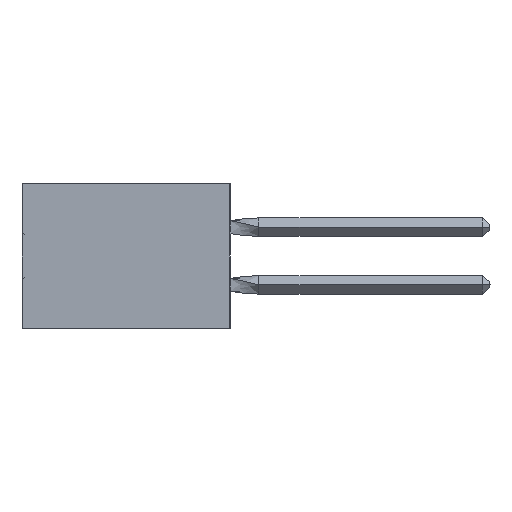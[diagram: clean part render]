
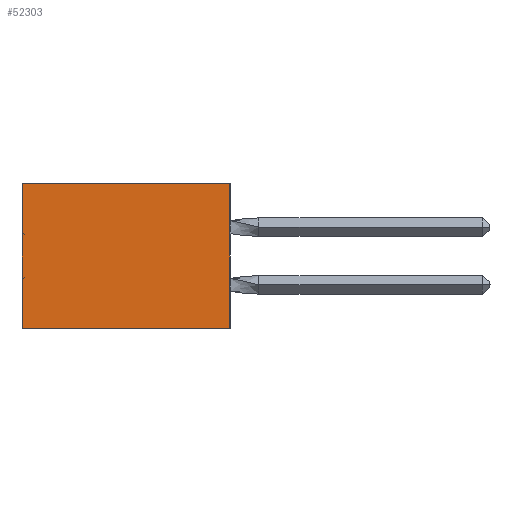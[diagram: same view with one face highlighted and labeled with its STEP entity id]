
A CAD part, left-side view. The second image highlights one B-rep face of the part: STEP entity #52303.
In plain terms, the highlighted planar face has unit normal (-1, 0, 0).
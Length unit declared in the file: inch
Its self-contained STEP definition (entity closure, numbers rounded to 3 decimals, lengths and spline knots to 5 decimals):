
#1045 = CARTESIAN_POINT ( 'NONE',  ( 0.305, 0., -0.5 ) ) ;
#2218 = ORIENTED_EDGE ( 'NONE', *, *, #22151, .T. ) ;
#2652 = FACE_OUTER_BOUND ( 'NONE', #12674, .T. ) ;
#3414 = ORIENTED_EDGE ( 'NONE', *, *, #12335, .F. ) ;
#4339 = EDGE_CURVE ( 'NONE', #31981, #32026, #5787, .T. ) ;
#4480 = LINE ( 'NONE', #23411, #48323 ) ;
#5787 = LINE ( 'NONE', #17353, #41653 ) ;
#7700 = VERTEX_POINT ( 'NONE', #12366 ) ;
#9683 = LINE ( 'NONE', #1045, #44156 ) ;
#11060 = CARTESIAN_POINT ( 'NONE',  ( 0.305, 0., -0.5 ) ) ;
#12187 = DIRECTION ( 'NONE',  ( 1., 0., 0. ) ) ;
#12335 = EDGE_CURVE ( 'NONE', #7700, #26019, #39653, .T. ) ;
#12366 = CARTESIAN_POINT ( 'NONE',  ( 0.305, 0., 0. ) ) ;
#12674 = EDGE_LOOP ( 'NONE', ( #26959, #19417, #3414, #2218 ) ) ;
#12756 = PLANE ( 'NONE',  #18285 ) ;
#17353 = CARTESIAN_POINT ( 'NONE',  ( 0.305, 0.72, -0.5 ) ) ;
#17668 = CARTESIAN_POINT ( 'NONE',  ( 0.305, 0.72, 0. ) ) ;
#18285 = AXIS2_PLACEMENT_3D ( 'NONE', #42452, #12187, #38009 ) ;
#19417 = ORIENTED_EDGE ( 'NONE', *, *, #46550, .F. ) ;
#22151 = EDGE_CURVE ( 'NONE', #7700, #31981, #4480, .T. ) ;
#23411 = CARTESIAN_POINT ( 'NONE',  ( 0.305, 0., 0. ) ) ;
#26019 = VERTEX_POINT ( 'NONE', #11060 ) ;
#26959 = ORIENTED_EDGE ( 'NONE', *, *, #4339, .T. ) ;
#31131 = DIRECTION ( 'NONE',  ( 0., 1., 0. ) ) ;
#31981 = VERTEX_POINT ( 'NONE', #17668 ) ;
#32026 = VERTEX_POINT ( 'NONE', #35929 ) ;
#35929 = CARTESIAN_POINT ( 'NONE',  ( 0.305, 0.72, -0.5 ) ) ;
#37259 = DIRECTION ( 'NONE',  ( 0., 0., -1. ) ) ;
#38009 = DIRECTION ( 'NONE',  ( 0., 0., -1. ) ) ;
#39653 = LINE ( 'NONE', #45962, #44252 ) ;
#41653 = VECTOR ( 'NONE', #51001, 39.37008 ) ;
#42452 = CARTESIAN_POINT ( 'NONE',  ( 0.305, 0., -0.5 ) ) ;
#44156 = VECTOR ( 'NONE', #31131, 39.37008 ) ;
#44252 = VECTOR ( 'NONE', #37259, 39.37008 ) ;
#44991 = DIRECTION ( 'NONE',  ( 0., 1., 0. ) ) ;
#45962 = CARTESIAN_POINT ( 'NONE',  ( 0.305, 0., -0.5 ) ) ;
#46550 = EDGE_CURVE ( 'NONE', #26019, #32026, #9683, .T. ) ;
#48323 = VECTOR ( 'NONE', #44991, 39.37008 ) ;
#51001 = DIRECTION ( 'NONE',  ( 0., 0., -1. ) ) ;
#52303 = ADVANCED_FACE ( 'NONE', ( #2652 ), #12756, .F. ) ;
